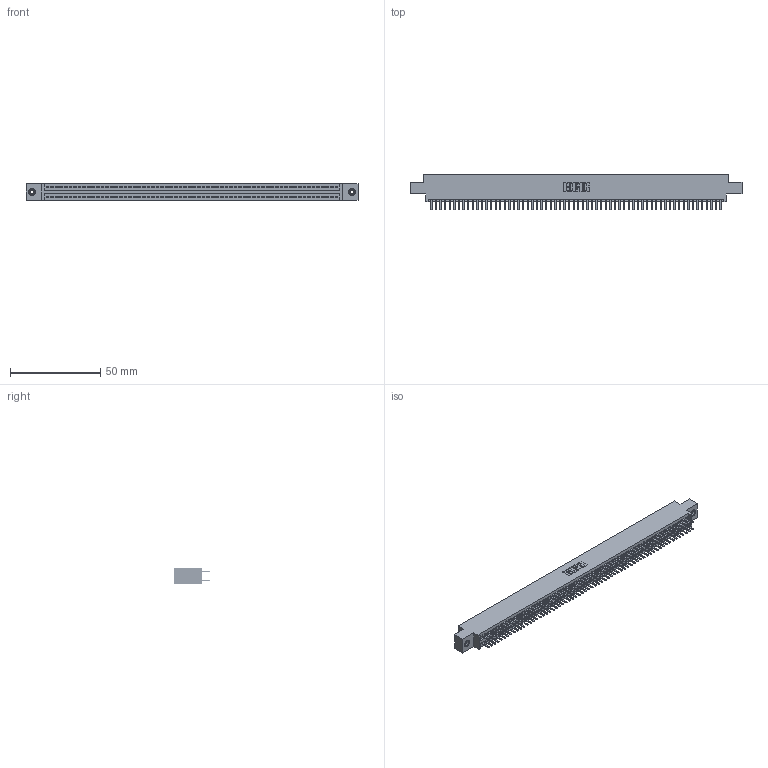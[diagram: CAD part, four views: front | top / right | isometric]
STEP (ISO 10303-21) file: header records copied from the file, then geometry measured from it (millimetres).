
FILE_DESCRIPTION (( 'STEP AP203' ), '1' );
FILE_NAME ('345-128-520-808.STEP', '2019-11-07T07:02:50', ( '' ), ( '' ), 'SwSTEP 2.0', 'SolidWorks 2016', '' );
FILE_SCHEMA (( 'CONFIG_CONTROL_DESIGN' ));
Length unit declared in the file: inch
Products named in the file (4): 345 Part_0.170 Offset - 0.156 Dia-TI; 345-292-001_345-293-120; 345-128-520-808; 345-250-001_345-250-003-102
Assembly tree (131 placements, depth 2):
  345-128-520-808
    345 Part_0.170 Offset - 0.156 Dia-TI
    345-292-001_345-293-120  x128
    345-250-001_345-250-003-102  x2
Bounding box: 183.77 x 19.68 x 9.4 mm (x, y, z)
Volume: 17879.5 mm3; surface area: 26892.3 mm2
Topology: 131 solids, 131 shells, 7102 faces, 20585 edges, 13374 vertices
Faces by surface type: plane 4596, cylinder 2490, cone 12, torus 4
Entity records: 48686 total; most frequent: CARTESIAN_POINT 8135, ORIENTED_EDGE 8050, DIRECTION 7159, EDGE_CURVE 4025, LINE 3613, VECTOR 3613, VERTEX_POINT 2676, AXIS2_PLACEMENT_3D 1773
